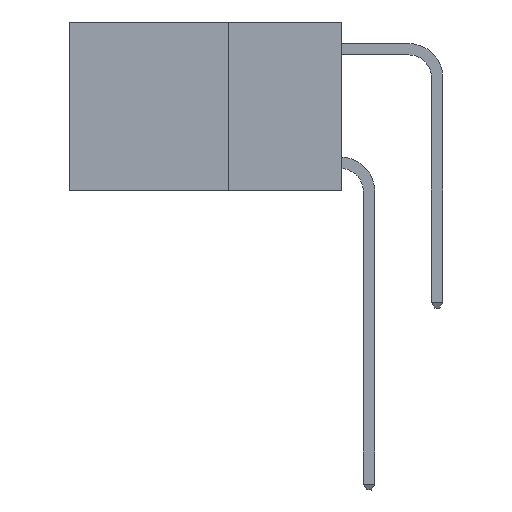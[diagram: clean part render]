
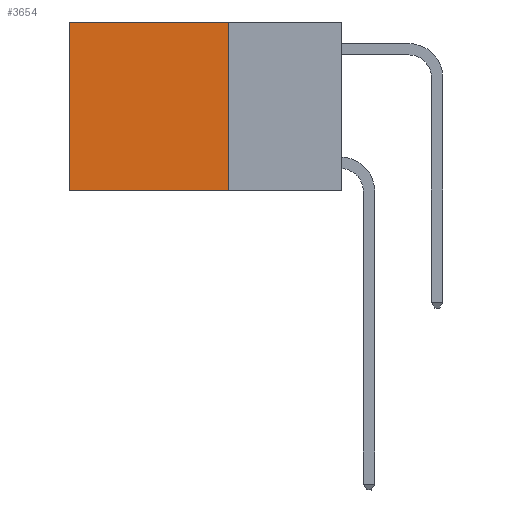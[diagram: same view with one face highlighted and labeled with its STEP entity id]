
A CAD part, left-side view. The second image highlights one B-rep face of the part: STEP entity #3654.
In plain terms, the highlighted planar face has unit normal (-1, 0, 0).
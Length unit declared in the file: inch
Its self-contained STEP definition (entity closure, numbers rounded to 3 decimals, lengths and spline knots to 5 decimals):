
#540 = EDGE_LOOP ( 'NONE', ( #3001, #707, #7660, #11239 ) ) ;
#707 = ORIENTED_EDGE ( 'NONE', *, *, #10269, .F. ) ;
#1184 = CARTESIAN_POINT ( 'NONE',  ( 0.2625, 0.25, 0. ) ) ;
#1576 = AXIS2_PLACEMENT_3D ( 'NONE', #3691, #7665, #1633 ) ;
#1633 = DIRECTION ( 'NONE',  ( 0., 0., -1. ) ) ;
#1872 = VECTOR ( 'NONE', #12166, 39.37008 ) ;
#2186 = EDGE_CURVE ( 'NONE', #4612, #5999, #7389, .T. ) ;
#2209 = CARTESIAN_POINT ( 'NONE',  ( 0.2625, 0.6, 0. ) ) ;
#2334 = DIRECTION ( 'NONE',  ( 0., 0., -1. ) ) ;
#2650 = CARTESIAN_POINT ( 'NONE',  ( 0.2625, 0.6, 0. ) ) ;
#3001 = ORIENTED_EDGE ( 'NONE', *, *, #2186, .T. ) ;
#3646 = CARTESIAN_POINT ( 'NONE',  ( 0.2625, 0.6, -0.37 ) ) ;
#3654 = ADVANCED_FACE ( 'NONE', ( #5036 ), #12456, .F. ) ;
#3691 = CARTESIAN_POINT ( 'NONE',  ( 0.2625, 0.25, 0. ) ) ;
#4240 = CARTESIAN_POINT ( 'NONE',  ( 0.2625, 0.25, 0. ) ) ;
#4612 = VERTEX_POINT ( 'NONE', #2209 ) ;
#4770 = VECTOR ( 'NONE', #2334, 39.37008 ) ;
#5036 = FACE_OUTER_BOUND ( 'NONE', #540, .T. ) ;
#5518 = VERTEX_POINT ( 'NONE', #8853 ) ;
#5999 = VERTEX_POINT ( 'NONE', #3646 ) ;
#6277 = DIRECTION ( 'NONE',  ( 0., 0., -1. ) ) ;
#6948 = LINE ( 'NONE', #11241, #1872 ) ;
#7349 = LINE ( 'NONE', #1184, #9654 ) ;
#7389 = LINE ( 'NONE', #2650, #4770 ) ;
#7660 = ORIENTED_EDGE ( 'NONE', *, *, #9865, .F. ) ;
#7665 = DIRECTION ( 'NONE',  ( 1., 0., 0. ) ) ;
#7844 = EDGE_CURVE ( 'NONE', #11513, #4612, #6948, .T. ) ;
#8853 = CARTESIAN_POINT ( 'NONE',  ( 0.2625, 0.25, -0.37 ) ) ;
#9654 = VECTOR ( 'NONE', #6277, 39.37008 ) ;
#9865 = EDGE_CURVE ( 'NONE', #11513, #5518, #7349, .T. ) ;
#10238 = VECTOR ( 'NONE', #10978, 39.37008 ) ;
#10269 = EDGE_CURVE ( 'NONE', #5518, #5999, #12740, .T. ) ;
#10978 = DIRECTION ( 'NONE',  ( 0., 1., 0. ) ) ;
#11239 = ORIENTED_EDGE ( 'NONE', *, *, #7844, .T. ) ;
#11241 = CARTESIAN_POINT ( 'NONE',  ( 0.2625, 0.25, 0. ) ) ;
#11513 = VERTEX_POINT ( 'NONE', #4240 ) ;
#11707 = CARTESIAN_POINT ( 'NONE',  ( 0.2625, 0.25, -0.37 ) ) ;
#12166 = DIRECTION ( 'NONE',  ( 0., 1., 0. ) ) ;
#12456 = PLANE ( 'NONE',  #1576 ) ;
#12740 = LINE ( 'NONE', #11707, #10238 ) ;
